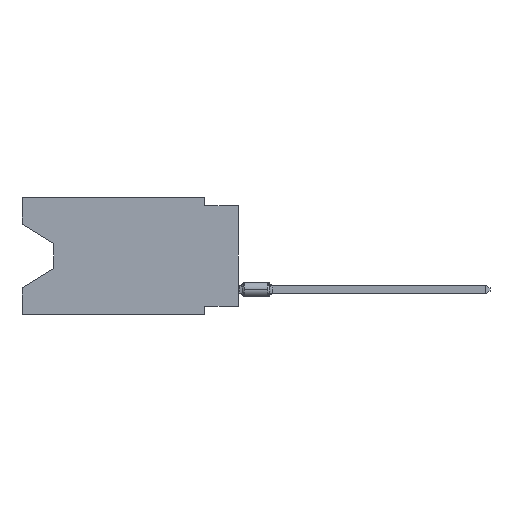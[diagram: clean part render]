
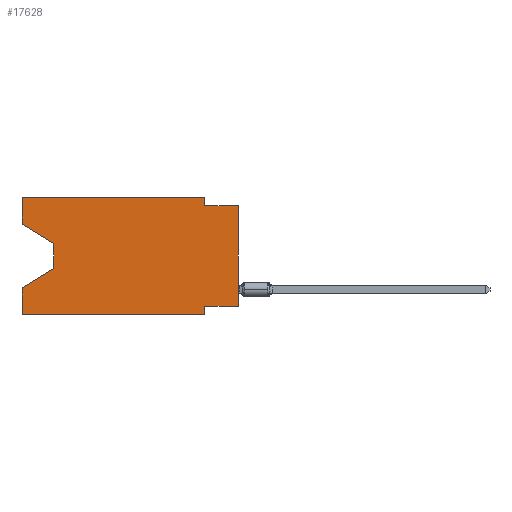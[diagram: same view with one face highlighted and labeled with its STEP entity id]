
A CAD part, left-side view. The second image highlights one B-rep face of the part: STEP entity #17628.
In plain terms, the highlighted planar face has unit normal (-1, 0, 0).
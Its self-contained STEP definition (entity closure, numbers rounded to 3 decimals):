
#391 = EDGE_CURVE ( 'NONE', #3130, #8962, #5386, .T. ) ;
#434 = EDGE_CURVE ( 'NONE', #2674, #13886, #15621, .T. ) ;
#609 = LINE ( 'NONE', #7410, #11359 ) ;
#661 = CARTESIAN_POINT ( 'NONE',  ( 0., 16.383, 0. ) ) ;
#710 = VECTOR ( 'NONE', #8686, 1000. ) ;
#783 = CARTESIAN_POINT ( 'NONE',  ( 0., 16.383, -6.852 ) ) ;
#912 = VERTEX_POINT ( 'NONE', #19863 ) ;
#1466 = DIRECTION ( 'NONE',  ( 0., 0., 1. ) ) ;
#1572 = CARTESIAN_POINT ( 'NONE',  ( 0., 0., 0. ) ) ;
#1897 = CARTESIAN_POINT ( 'NONE',  ( 0., 2.54, 0. ) ) ;
#2476 = DIRECTION ( 'NONE',  ( 0., -1., 0. ) ) ;
#2674 = VERTEX_POINT ( 'NONE', #15514 ) ;
#2997 = VECTOR ( 'NONE', #7218, 1000. ) ;
#3130 = VERTEX_POINT ( 'NONE', #20466 ) ;
#3515 = AXIS2_PLACEMENT_3D ( 'NONE', #8346, #15381, #18899 ) ;
#4162 = VERTEX_POINT ( 'NONE', #15643 ) ;
#4218 = CARTESIAN_POINT ( 'NONE',  ( 0., 2.54, -8.255 ) ) ;
#4223 = CARTESIAN_POINT ( 'NONE',  ( 0., 2.54, -0.635 ) ) ;
#4254 = CARTESIAN_POINT ( 'NONE',  ( 0., 16.383, -8.89 ) ) ;
#4266 = EDGE_CURVE ( 'NONE', #2674, #7038, #22252, .T. ) ;
#4354 = VERTEX_POINT ( 'NONE', #14493 ) ;
#4808 = LINE ( 'NONE', #16610, #19156 ) ;
#5340 = EDGE_CURVE ( 'NONE', #16824, #5802, #13631, .T. ) ;
#5386 = LINE ( 'NONE', #22440, #710 ) ;
#5436 = VECTOR ( 'NONE', #20544, 1000. ) ;
#5595 = DIRECTION ( 'NONE',  ( 0., 0., -1. ) ) ;
#5694 = CARTESIAN_POINT ( 'NONE',  ( 0., 0., -0.635 ) ) ;
#5707 = VECTOR ( 'NONE', #19051, 1000. ) ;
#5802 = VERTEX_POINT ( 'NONE', #16339 ) ;
#5858 = EDGE_LOOP ( 'NONE', ( #20582, #19539, #18023, #9069, #18531, #18617, #7886, #6524, #19868, #19947, #6923, #21346 ) ) ;
#6102 = LINE ( 'NONE', #661, #11333 ) ;
#6120 = VECTOR ( 'NONE', #16356, 1000. ) ;
#6524 = ORIENTED_EDGE ( 'NONE', *, *, #434, .T. ) ;
#6923 = ORIENTED_EDGE ( 'NONE', *, *, #9582, .F. ) ;
#7038 = VERTEX_POINT ( 'NONE', #4218 ) ;
#7218 = DIRECTION ( 'NONE',  ( 0., -1., 0. ) ) ;
#7410 = CARTESIAN_POINT ( 'NONE',  ( 0., 13.97, -3.505 ) ) ;
#7886 = ORIENTED_EDGE ( 'NONE', *, *, #4266, .F. ) ;
#7913 = VECTOR ( 'NONE', #10690, 1000. ) ;
#8196 = CARTESIAN_POINT ( 'NONE',  ( 0., 16.383, -2.038 ) ) ;
#8198 = VERTEX_POINT ( 'NONE', #11056 ) ;
#8202 = EDGE_CURVE ( 'NONE', #8198, #4162, #19806, .T. ) ;
#8346 = CARTESIAN_POINT ( 'NONE',  ( 0., 16.383, 0. ) ) ;
#8686 = DIRECTION ( 'NONE',  ( 0., 0.855, -0.519 ) ) ;
#8939 = VECTOR ( 'NONE', #21070, 1000. ) ;
#8962 = VERTEX_POINT ( 'NONE', #783 ) ;
#9069 = ORIENTED_EDGE ( 'NONE', *, *, #20902, .F. ) ;
#9582 = EDGE_CURVE ( 'NONE', #4354, #912, #6102, .T. ) ;
#10469 = VECTOR ( 'NONE', #1466, 1000. ) ;
#10627 = CARTESIAN_POINT ( 'NONE',  ( 0., 0., -0.635 ) ) ;
#10690 = DIRECTION ( 'NONE',  ( 0., 0., -1. ) ) ;
#10699 = VERTEX_POINT ( 'NONE', #4223 ) ;
#11027 = LINE ( 'NONE', #19776, #7913 ) ;
#11056 = CARTESIAN_POINT ( 'NONE',  ( 0., 16.383, -8.89 ) ) ;
#11328 = EDGE_CURVE ( 'NONE', #10699, #13886, #13612, .T. ) ;
#11333 = VECTOR ( 'NONE', #2476, 1000. ) ;
#11359 = VECTOR ( 'NONE', #5595, 1000. ) ;
#13408 = DIRECTION ( 'NONE',  ( 0., -0.855, -0.519 ) ) ;
#13612 = LINE ( 'NONE', #10627, #5436 ) ;
#13631 = LINE ( 'NONE', #8196, #13951 ) ;
#13819 = CARTESIAN_POINT ( 'NONE',  ( 0., 0., -8.255 ) ) ;
#13886 = VERTEX_POINT ( 'NONE', #5694 ) ;
#13951 = VECTOR ( 'NONE', #13408, 1000. ) ;
#14250 = LINE ( 'NONE', #1897, #8939 ) ;
#14493 = CARTESIAN_POINT ( 'NONE',  ( 0., 16.383, 0. ) ) ;
#15381 = DIRECTION ( 'NONE',  ( 1., 0., 0. ) ) ;
#15514 = CARTESIAN_POINT ( 'NONE',  ( 0., 0., -8.255 ) ) ;
#15621 = LINE ( 'NONE', #1572, #10469 ) ;
#15643 = CARTESIAN_POINT ( 'NONE',  ( 0., 2.54, -8.89 ) ) ;
#16187 = EDGE_CURVE ( 'NONE', #5802, #3130, #609, .T. ) ;
#16339 = CARTESIAN_POINT ( 'NONE',  ( 0., 13.97, -3.505 ) ) ;
#16356 = DIRECTION ( 'NONE',  ( 0., 0., 1. ) ) ;
#16586 = CARTESIAN_POINT ( 'NONE',  ( 0., 16.383, -2.038 ) ) ;
#16610 = CARTESIAN_POINT ( 'NONE',  ( 0., 16.383, 0. ) ) ;
#16824 = VERTEX_POINT ( 'NONE', #16586 ) ;
#17478 = EDGE_CURVE ( 'NONE', #912, #10699, #14250, .T. ) ;
#17523 = PLANE ( 'NONE',  #3515 ) ;
#17628 = ADVANCED_FACE ( 'NONE', ( #20916 ), #17523, .F. ) ;
#17719 = CARTESIAN_POINT ( 'NONE',  ( 0., 16.383, 0. ) ) ;
#17949 = LINE ( 'NONE', #17719, #6120 ) ;
#18023 = ORIENTED_EDGE ( 'NONE', *, *, #391, .T. ) ;
#18531 = ORIENTED_EDGE ( 'NONE', *, *, #8202, .T. ) ;
#18617 = ORIENTED_EDGE ( 'NONE', *, *, #19287, .F. ) ;
#18899 = DIRECTION ( 'NONE',  ( 0., 0., -1. ) ) ;
#19051 = DIRECTION ( 'NONE',  ( 0., 1., 0. ) ) ;
#19156 = VECTOR ( 'NONE', #20013, 1000. ) ;
#19287 = EDGE_CURVE ( 'NONE', #7038, #4162, #11027, .T. ) ;
#19539 = ORIENTED_EDGE ( 'NONE', *, *, #16187, .T. ) ;
#19776 = CARTESIAN_POINT ( 'NONE',  ( 0., 2.54, -8.89 ) ) ;
#19806 = LINE ( 'NONE', #4254, #2997 ) ;
#19863 = CARTESIAN_POINT ( 'NONE',  ( 0., 2.54, 0. ) ) ;
#19868 = ORIENTED_EDGE ( 'NONE', *, *, #11328, .F. ) ;
#19947 = ORIENTED_EDGE ( 'NONE', *, *, #17478, .F. ) ;
#20013 = DIRECTION ( 'NONE',  ( 0., 0., 1. ) ) ;
#20466 = CARTESIAN_POINT ( 'NONE',  ( 0., 13.97, -5.385 ) ) ;
#20544 = DIRECTION ( 'NONE',  ( 0., -1., 0. ) ) ;
#20582 = ORIENTED_EDGE ( 'NONE', *, *, #5340, .T. ) ;
#20639 = EDGE_CURVE ( 'NONE', #16824, #4354, #4808, .T. ) ;
#20902 = EDGE_CURVE ( 'NONE', #8198, #8962, #17949, .T. ) ;
#20916 = FACE_OUTER_BOUND ( 'NONE', #5858, .T. ) ;
#21070 = DIRECTION ( 'NONE',  ( 0., 0., -1. ) ) ;
#21346 = ORIENTED_EDGE ( 'NONE', *, *, #20639, .F. ) ;
#22252 = LINE ( 'NONE', #13819, #5707 ) ;
#22440 = CARTESIAN_POINT ( 'NONE',  ( 0., 13.97, -5.385 ) ) ;
